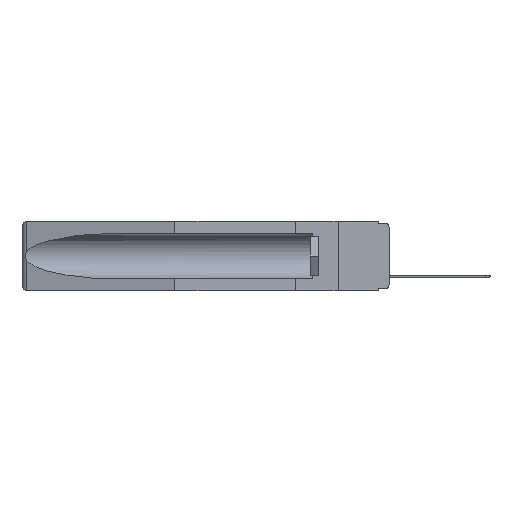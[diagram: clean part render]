
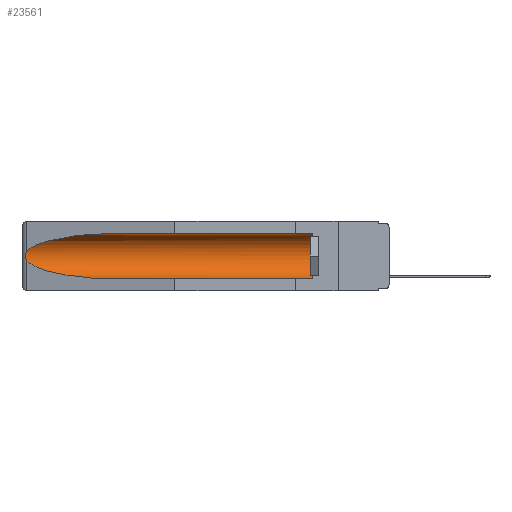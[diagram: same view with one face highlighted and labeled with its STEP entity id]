
A CAD part, left-side view. The second image highlights one B-rep face of the part: STEP entity #23561.
In plain terms, the highlighted cylindrical face has radius 2.857 mm (diameter 5.715 mm), a partial arc.
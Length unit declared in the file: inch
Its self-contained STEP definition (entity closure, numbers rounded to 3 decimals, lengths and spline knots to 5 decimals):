
#592 = AXIS2_PLACEMENT_3D ( 'NONE', #5821, #5426, #23270 ) ;
#621 = CARTESIAN_POINT ( 'NONE',  ( 0.25451, 1.48313, -0.24835 ) ) ;
#973 = CARTESIAN_POINT ( 'NONE',  ( 0.155, 1.07973, -0.059 ) ) ;
#1368 = CARTESIAN_POINT ( 'NONE',  ( 0.26537, 1.52718, -0.14972 ) ) ;
#1590 = DIRECTION ( 'NONE',  ( 0., 0., 1. ) ) ;
#1651 = CARTESIAN_POINT ( 'NONE',  ( 0.26597, 1.52961, -0.15275 ) ) ;
#2085 = ORIENTED_EDGE ( 'NONE', *, *, #18471, .T. ) ;
#2256 = CARTESIAN_POINT ( 'NONE',  ( 0.26537, 1.52718, -0.14972 ) ) ;
#3200 = ORIENTED_EDGE ( 'NONE', *, *, #11199, .T. ) ;
#4225 = DIRECTION ( 'NONE',  ( 0., 1., 0. ) ) ;
#4549 = ORIENTED_EDGE ( 'NONE', *, *, #21394, .T. ) ;
#5032 = VERTEX_POINT ( 'NONE', #12430 ) ;
#5349 = CARTESIAN_POINT ( 'NONE',  ( 0.26597, 1.5296, -0.19026 ) ) ;
#5426 = DIRECTION ( 'NONE',  ( 0., -1., 0. ) ) ;
#5593 = CARTESIAN_POINT ( 'NONE',  ( 0.2675, 1.53308, -0.16763 ) ) ;
#5821 = CARTESIAN_POINT ( 'NONE',  ( 0.155, 0.126, -0.1715 ) ) ;
#6355 = EDGE_LOOP ( 'NONE', ( #7624, #4549, #2085, #17555, #3200, #17304 ) ) ;
#6461 = B_SPLINE_CURVE_WITH_KNOTS ( 'NONE', 3,
 ( #11360, #1651, #19122, #7175, #5593, #17143, #21612, #23583, #5349, #25156 ),
 .UNSPECIFIED., .F., .F.,
 ( 4, 2, 2, 2, 4 ),
 ( 0., 0.00029, 0.00058, 0.00087, 0.00117 ),
 .UNSPECIFIED. ) ;
#6554 = CARTESIAN_POINT ( 'NONE',  ( 0.21114, 1.30732, -0.284 ) ) ;
#7025 = VERTEX_POINT ( 'NONE', #19729 ) ;
#7031 = VECTOR ( 'NONE', #24898, 39.37008 ) ;
#7175 = CARTESIAN_POINT ( 'NONE',  ( 0.2673, 1.5327, -0.16383 ) ) ;
#7624 = ORIENTED_EDGE ( 'NONE', *, *, #14464, .T. ) ;
#7900 = CARTESIAN_POINT ( 'NONE',  ( 0.155, 1.07973, -0.284 ) ) ;
#8596 =( BOUNDED_CURVE ( )  B_SPLINE_CURVE ( 3, ( #18484, #621, #6554, #20471 ),
 .UNSPECIFIED., .F., .T. ) 
 B_SPLINE_CURVE_WITH_KNOTS ( ( 4, 4 ),
 ( 0.1948, 1.5708 ),
 .UNSPECIFIED. ) 
 CURVE ( )  GEOMETRIC_REPRESENTATION_ITEM ( )  RATIONAL_B_SPLINE_CURVE ( ( 1., 0.848, 0.848, 1. ) ) 
 REPRESENTATION_ITEM ( '' )  );
#8748 =( BOUNDED_CURVE ( )  B_SPLINE_CURVE ( 3, ( #973, #11076, #25149, #1368 ),
 .UNSPECIFIED., .F., .T. ) 
 B_SPLINE_CURVE_WITH_KNOTS ( ( 4, 4 ),
 ( 4.71239, 6.08839 ),
 .UNSPECIFIED. ) 
 CURVE ( )  GEOMETRIC_REPRESENTATION_ITEM ( )  RATIONAL_B_SPLINE_CURVE ( ( 1., 0.848, 0.848, 1. ) ) 
 REPRESENTATION_ITEM ( '' )  );
#9455 = FACE_OUTER_BOUND ( 'NONE', #6355, .T. ) ;
#9844 = LINE ( 'NONE', #16876, #7031 ) ;
#11076 = CARTESIAN_POINT ( 'NONE',  ( 0.21114, 1.30732, -0.059 ) ) ;
#11199 = EDGE_CURVE ( 'NONE', #13178, #7025, #19894, .T. ) ;
#11360 = CARTESIAN_POINT ( 'NONE',  ( 0.26537, 1.52718, -0.14972 ) ) ;
#12430 = CARTESIAN_POINT ( 'NONE',  ( 0.155, 1.07973, -0.059 ) ) ;
#13178 = VERTEX_POINT ( 'NONE', #25240 ) ;
#13526 = CYLINDRICAL_SURFACE ( 'NONE', #24554, 0.1125 ) ;
#14464 = EDGE_CURVE ( 'NONE', #5032, #17459, #8748, .T. ) ;
#14908 = VECTOR ( 'NONE', #4225, 39.37008 ) ;
#16637 = VERTEX_POINT ( 'NONE', #7900 ) ;
#16876 = CARTESIAN_POINT ( 'NONE',  ( 0.155, -0.30754, -0.059 ) ) ;
#17143 = CARTESIAN_POINT ( 'NONE',  ( 0.2675, 1.53308, -0.17534 ) ) ;
#17213 = DIRECTION ( 'NONE',  ( 0., 1., 0. ) ) ;
#17304 = ORIENTED_EDGE ( 'NONE', *, *, #25628, .T. ) ;
#17459 = VERTEX_POINT ( 'NONE', #2256 ) ;
#17555 = ORIENTED_EDGE ( 'NONE', *, *, #20882, .F. ) ;
#18471 = EDGE_CURVE ( 'NONE', #20968, #16637, #8596, .T. ) ;
#18484 = CARTESIAN_POINT ( 'NONE',  ( 0.26537, 1.52718, -0.19328 ) ) ;
#18666 = CARTESIAN_POINT ( 'NONE',  ( 0.155, -0.30754, -0.284 ) ) ;
#19122 = CARTESIAN_POINT ( 'NONE',  ( 0.26654, 1.53092, -0.15636 ) ) ;
#19729 = CARTESIAN_POINT ( 'NONE',  ( 0.155, 0.126, -0.059 ) ) ;
#19894 = CIRCLE ( 'NONE', #592, 0.1125 ) ;
#20471 = CARTESIAN_POINT ( 'NONE',  ( 0.155, 1.07973, -0.284 ) ) ;
#20882 = EDGE_CURVE ( 'NONE', #13178, #16637, #22345, .T. ) ;
#20968 = VERTEX_POINT ( 'NONE', #23359 ) ;
#21394 = EDGE_CURVE ( 'NONE', #17459, #20968, #6461, .T. ) ;
#21612 = CARTESIAN_POINT ( 'NONE',  ( 0.2673, 1.53269, -0.17917 ) ) ;
#22345 = LINE ( 'NONE', #18666, #14908 ) ;
#23262 = CARTESIAN_POINT ( 'NONE',  ( 0.155, -0.30754, -0.1715 ) ) ;
#23270 = DIRECTION ( 'NONE',  ( 0., 0., 1. ) ) ;
#23359 = CARTESIAN_POINT ( 'NONE',  ( 0.26537, 1.52718, -0.19328 ) ) ;
#23561 = ADVANCED_FACE ( 'NONE', ( #9455 ), #13526, .F. ) ;
#23583 = CARTESIAN_POINT ( 'NONE',  ( 0.26655, 1.53094, -0.18657 ) ) ;
#24554 = AXIS2_PLACEMENT_3D ( 'NONE', #23262, #17213, #1590 ) ;
#24898 = DIRECTION ( 'NONE',  ( 0., 1., 0. ) ) ;
#25149 = CARTESIAN_POINT ( 'NONE',  ( 0.25451, 1.48313, -0.09465 ) ) ;
#25156 = CARTESIAN_POINT ( 'NONE',  ( 0.26537, 1.52718, -0.19328 ) ) ;
#25240 = CARTESIAN_POINT ( 'NONE',  ( 0.155, 0.126, -0.284 ) ) ;
#25628 = EDGE_CURVE ( 'NONE', #7025, #5032, #9844, .T. ) ;
